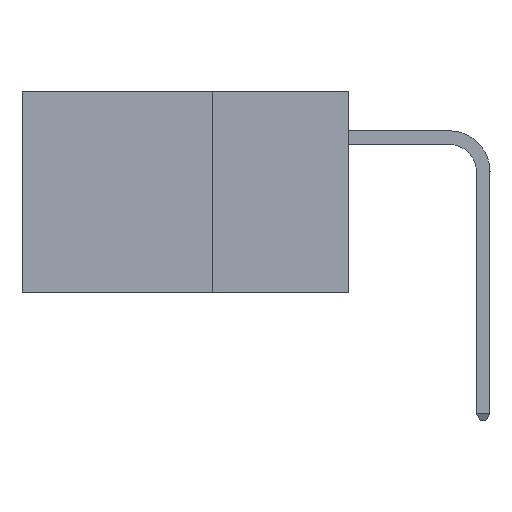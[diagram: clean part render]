
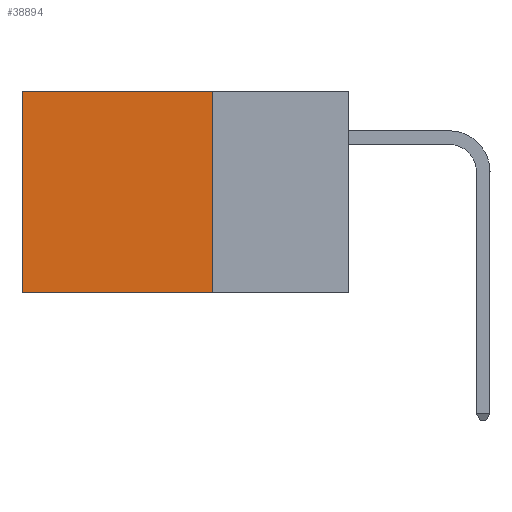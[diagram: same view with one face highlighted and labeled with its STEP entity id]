
A CAD part, left-side view. The second image highlights one B-rep face of the part: STEP entity #38894.
In plain terms, the highlighted planar face has unit normal (-1, 0, 0).
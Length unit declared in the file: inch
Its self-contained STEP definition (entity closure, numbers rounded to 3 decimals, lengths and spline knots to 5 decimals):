
#54 = VERTEX_POINT ( 'NONE', #20230 ) ;
#1074 = PLANE ( 'NONE',  #19260 ) ;
#3287 = CARTESIAN_POINT ( 'NONE',  ( 0.2875, 0.25, 0. ) ) ;
#4798 = DIRECTION ( 'NONE',  ( 0., 0., -1. ) ) ;
#8830 = ORIENTED_EDGE ( 'NONE', *, *, #43045, .T. ) ;
#11066 = LINE ( 'NONE', #22232, #12772 ) ;
#12772 = VECTOR ( 'NONE', #36694, 39.37008 ) ;
#14824 = ORIENTED_EDGE ( 'NONE', *, *, #25437, .T. ) ;
#15155 = CARTESIAN_POINT ( 'NONE',  ( 0.2875, 0.25, -0.37 ) ) ;
#15654 = VECTOR ( 'NONE', #45889, 39.37008 ) ;
#15815 = CARTESIAN_POINT ( 'NONE',  ( 0.2875, 0.25, 0. ) ) ;
#16938 = LINE ( 'NONE', #15815, #21561 ) ;
#17799 = DIRECTION ( 'NONE',  ( 0., 1., 0. ) ) ;
#19260 = AXIS2_PLACEMENT_3D ( 'NONE', #45208, #34281, #4798 ) ;
#20024 = FACE_OUTER_BOUND ( 'NONE', #47325, .T. ) ;
#20230 = CARTESIAN_POINT ( 'NONE',  ( 0.2875, 0.6, 0. ) ) ;
#21561 = VECTOR ( 'NONE', #30590, 39.37008 ) ;
#21568 = VERTEX_POINT ( 'NONE', #28320 ) ;
#22132 = ORIENTED_EDGE ( 'NONE', *, *, #26275, .F. ) ;
#22232 = CARTESIAN_POINT ( 'NONE',  ( 0.2875, 0.25, -0.37 ) ) ;
#23542 = CARTESIAN_POINT ( 'NONE',  ( 0.2875, 0.6, 0. ) ) ;
#25437 = EDGE_CURVE ( 'NONE', #44595, #54, #26246, .T. ) ;
#26246 = LINE ( 'NONE', #32425, #29103 ) ;
#26275 = EDGE_CURVE ( 'NONE', #44595, #35426, #16938, .T. ) ;
#28320 = CARTESIAN_POINT ( 'NONE',  ( 0.2875, 0.6, -0.37 ) ) ;
#29103 = VECTOR ( 'NONE', #17799, 39.37008 ) ;
#30590 = DIRECTION ( 'NONE',  ( 0., 0., -1. ) ) ;
#32425 = CARTESIAN_POINT ( 'NONE',  ( 0.2875, 0.25, 0. ) ) ;
#34281 = DIRECTION ( 'NONE',  ( 1., 0., 0. ) ) ;
#34433 = ORIENTED_EDGE ( 'NONE', *, *, #43400, .F. ) ;
#35426 = VERTEX_POINT ( 'NONE', #15155 ) ;
#36694 = DIRECTION ( 'NONE',  ( 0., 1., 0. ) ) ;
#38894 = ADVANCED_FACE ( 'NONE', ( #20024 ), #1074, .F. ) ;
#42150 = LINE ( 'NONE', #23542, #15654 ) ;
#43045 = EDGE_CURVE ( 'NONE', #54, #21568, #42150, .T. ) ;
#43400 = EDGE_CURVE ( 'NONE', #35426, #21568, #11066, .T. ) ;
#44595 = VERTEX_POINT ( 'NONE', #3287 ) ;
#45208 = CARTESIAN_POINT ( 'NONE',  ( 0.2875, 0.25, 0. ) ) ;
#45889 = DIRECTION ( 'NONE',  ( 0., 0., -1. ) ) ;
#47325 = EDGE_LOOP ( 'NONE', ( #8830, #34433, #22132, #14824 ) ) ;
